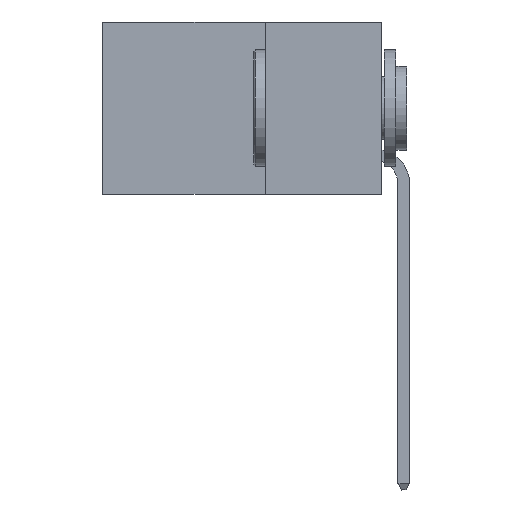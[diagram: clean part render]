
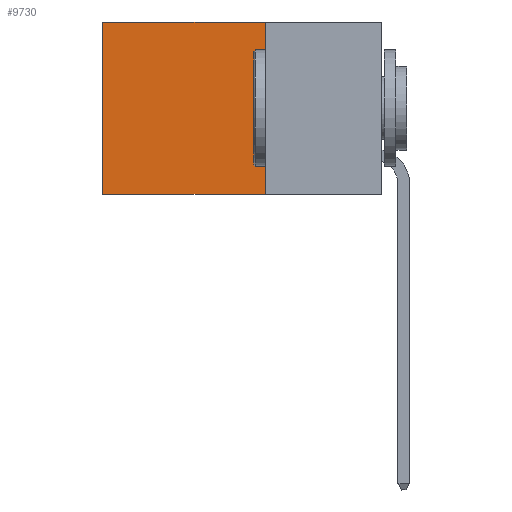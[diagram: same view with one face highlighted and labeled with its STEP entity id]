
A CAD part, left-side view. The second image highlights one B-rep face of the part: STEP entity #9730.
In plain terms, the highlighted planar face has unit normal (-1, 0, 0).
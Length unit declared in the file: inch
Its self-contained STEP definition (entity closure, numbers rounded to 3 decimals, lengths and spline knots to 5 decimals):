
#900 = CARTESIAN_POINT ( 'NONE',  ( 0.2875, 0.25, 0. ) ) ;
#1301 = VECTOR ( 'NONE', #5107, 39.37008 ) ;
#1667 = LINE ( 'NONE', #26836, #22001 ) ;
#2156 = ORIENTED_EDGE ( 'NONE', *, *, #14983, .T. ) ;
#4109 = EDGE_CURVE ( 'NONE', #19812, #24531, #1667, .T. ) ;
#4330 = ORIENTED_EDGE ( 'NONE', *, *, #4109, .F. ) ;
#4381 = CARTESIAN_POINT ( 'NONE',  ( 0.2875, 0.25, 0. ) ) ;
#4391 = LINE ( 'NONE', #29666, #1301 ) ;
#4671 = EDGE_CURVE ( 'NONE', #24531, #15932, #16129, .T. ) ;
#5107 = DIRECTION ( 'NONE',  ( 0., 1., 0. ) ) ;
#7662 = CARTESIAN_POINT ( 'NONE',  ( 0.2875, 0.25, -0.37 ) ) ;
#8218 = PLANE ( 'NONE',  #30968 ) ;
#8679 = EDGE_LOOP ( 'NONE', ( #21451, #22613, #4330, #2156 ) ) ;
#9274 = FACE_OUTER_BOUND ( 'NONE', #8679, .T. ) ;
#9730 = ADVANCED_FACE ( 'NONE', ( #9274 ), #8218, .F. ) ;
#12569 = CARTESIAN_POINT ( 'NONE',  ( 0.2875, 0.25, -0.37 ) ) ;
#14983 = EDGE_CURVE ( 'NONE', #19812, #15850, #4391, .T. ) ;
#15678 = DIRECTION ( 'NONE',  ( 0., 1., 0. ) ) ;
#15850 = VERTEX_POINT ( 'NONE', #22180 ) ;
#15932 = VERTEX_POINT ( 'NONE', #17732 ) ;
#16129 = LINE ( 'NONE', #12569, #21132 ) ;
#17732 = CARTESIAN_POINT ( 'NONE',  ( 0.2875, 0.6, -0.37 ) ) ;
#17931 = CARTESIAN_POINT ( 'NONE',  ( 0.2875, 0.6, 0. ) ) ;
#18304 = DIRECTION ( 'NONE',  ( 1., 0., 0. ) ) ;
#19812 = VERTEX_POINT ( 'NONE', #4381 ) ;
#21132 = VECTOR ( 'NONE', #15678, 39.37008 ) ;
#21451 = ORIENTED_EDGE ( 'NONE', *, *, #29426, .T. ) ;
#22001 = VECTOR ( 'NONE', #31517, 39.37008 ) ;
#22180 = CARTESIAN_POINT ( 'NONE',  ( 0.2875, 0.6, 0. ) ) ;
#22613 = ORIENTED_EDGE ( 'NONE', *, *, #4671, .F. ) ;
#23005 = DIRECTION ( 'NONE',  ( 0., 0., -1. ) ) ;
#24531 = VERTEX_POINT ( 'NONE', #7662 ) ;
#25647 = DIRECTION ( 'NONE',  ( 0., 0., -1. ) ) ;
#26002 = VECTOR ( 'NONE', #25647, 39.37008 ) ;
#26836 = CARTESIAN_POINT ( 'NONE',  ( 0.2875, 0.25, 0. ) ) ;
#27511 = LINE ( 'NONE', #17931, #26002 ) ;
#29426 = EDGE_CURVE ( 'NONE', #15850, #15932, #27511, .T. ) ;
#29666 = CARTESIAN_POINT ( 'NONE',  ( 0.2875, 0.25, 0. ) ) ;
#30968 = AXIS2_PLACEMENT_3D ( 'NONE', #900, #18304, #23005 ) ;
#31517 = DIRECTION ( 'NONE',  ( 0., 0., -1. ) ) ;
